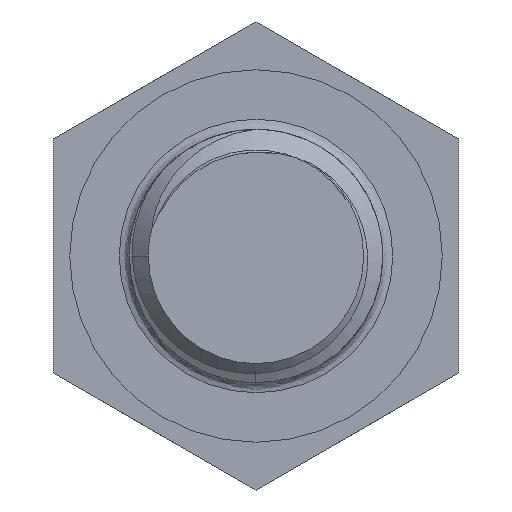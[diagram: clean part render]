
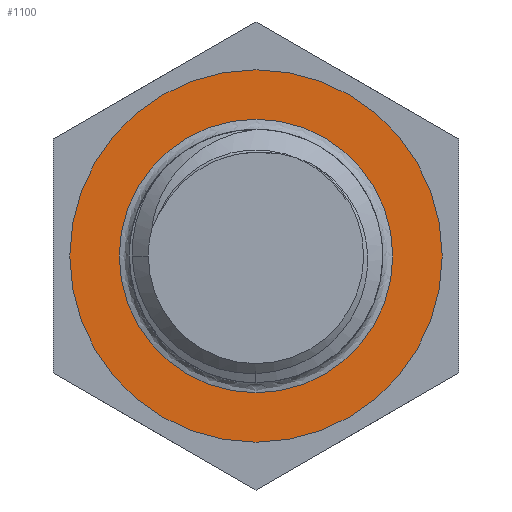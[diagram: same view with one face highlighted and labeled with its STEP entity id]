
A CAD part, left-side view. The second image highlights one B-rep face of the part: STEP entity #1100.
In plain terms, the highlighted planar face has unit normal (-1, 0, 0).
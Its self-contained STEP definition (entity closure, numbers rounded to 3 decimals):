
#817 = CYLINDRICAL_SURFACE('',#818,7.35);
#818 = AXIS2_PLACEMENT_3D('',#819,#820,#821);
#819 = CARTESIAN_POINT('',(-6.7,0.,0.));
#820 = DIRECTION('',(-1.,-0.,0.));
#821 = DIRECTION('',(0.,0.,-1.));
#1051 = VERTEX_POINT('',#1052);
#1052 = CARTESIAN_POINT('',(-7.,0.,-7.35));
#1073 = EDGE_CURVE('',#1051,#1051,#1074,.T.);
#1074 = SURFACE_CURVE('',#1075,(#1080,#1087),.PCURVE_S1.);
#1075 = CIRCLE('',#1076,7.35);
#1076 = AXIS2_PLACEMENT_3D('',#1077,#1078,#1079);
#1077 = CARTESIAN_POINT('',(-7.,0.,0.));
#1078 = DIRECTION('',(1.,-0.,0.));
#1079 = DIRECTION('',(0.,0.,-1.));
#1080 = PCURVE('',#817,#1081);
#1081 = DEFINITIONAL_REPRESENTATION('',(#1082),#1086);
#1082 = LINE('',#1083,#1084);
#1083 = CARTESIAN_POINT('',(-0.,0.3));
#1084 = VECTOR('',#1085,1.);
#1085 = DIRECTION('',(-1.,0.));
#1086 = ( GEOMETRIC_REPRESENTATION_CONTEXT(2) 
PARAMETRIC_REPRESENTATION_CONTEXT() REPRESENTATION_CONTEXT('2D SPACE',''
  ) );
#1087 = PCURVE('',#1088,#1093);
#1088 = PLANE('',#1089);
#1089 = AXIS2_PLACEMENT_3D('',#1090,#1091,#1092);
#1090 = CARTESIAN_POINT('',(-7.,0.,0.));
#1091 = DIRECTION('',(1.,0.,0.));
#1092 = DIRECTION('',(0.,0.,-1.));
#1093 = DEFINITIONAL_REPRESENTATION('',(#1094),#1098);
#1094 = CIRCLE('',#1095,7.35);
#1095 = AXIS2_PLACEMENT_2D('',#1096,#1097);
#1096 = CARTESIAN_POINT('',(0.,0.));
#1097 = DIRECTION('',(1.,0.));
#1098 = ( GEOMETRIC_REPRESENTATION_CONTEXT(2) 
PARAMETRIC_REPRESENTATION_CONTEXT() REPRESENTATION_CONTEXT('2D SPACE',''
  ) );
#1100 = ADVANCED_FACE('',(#1101,#1104),#1088,.F.);
#1101 = FACE_BOUND('',#1102,.F.);
#1102 = EDGE_LOOP('',(#1103));
#1103 = ORIENTED_EDGE('',*,*,#1073,.T.);
#1104 = FACE_BOUND('',#1105,.F.);
#1105 = EDGE_LOOP('',(#1106));
#1106 = ORIENTED_EDGE('',*,*,#1107,.F.);
#1107 = EDGE_CURVE('',#1108,#1108,#1110,.T.);
#1108 = VERTEX_POINT('',#1109);
#1109 = CARTESIAN_POINT('',(-7.,0.,-5.4));
#1110 = SURFACE_CURVE('',#1111,(#1116,#1123),.PCURVE_S1.);
#1111 = CIRCLE('',#1112,5.4);
#1112 = AXIS2_PLACEMENT_3D('',#1113,#1114,#1115);
#1113 = CARTESIAN_POINT('',(-7.,0.,0.));
#1114 = DIRECTION('',(1.,-0.,0.));
#1115 = DIRECTION('',(0.,0.,-1.));
#1116 = PCURVE('',#1088,#1117);
#1117 = DEFINITIONAL_REPRESENTATION('',(#1118),#1122);
#1118 = CIRCLE('',#1119,5.4);
#1119 = AXIS2_PLACEMENT_2D('',#1120,#1121);
#1120 = CARTESIAN_POINT('',(0.,0.));
#1121 = DIRECTION('',(1.,0.));
#1122 = ( GEOMETRIC_REPRESENTATION_CONTEXT(2) 
PARAMETRIC_REPRESENTATION_CONTEXT() REPRESENTATION_CONTEXT('2D SPACE',''
  ) );
#1123 = PCURVE('',#1124,#1133);
#1124 = SURFACE_OF_REVOLUTION('',#1125,#1130);
#1125 = CIRCLE('',#1126,0.4);
#1126 = AXIS2_PLACEMENT_3D('',#1127,#1128,#1129);
#1127 = CARTESIAN_POINT('',(-7.4,0.,-5.4));
#1128 = DIRECTION('',(0.,-1.,0.));
#1129 = DIRECTION('',(1.,0.,0.));
#1130 = AXIS1_PLACEMENT('',#1131,#1132);
#1131 = CARTESIAN_POINT('',(-7.,0.,0.));
#1132 = DIRECTION('',(1.,0.,0.));
#1133 = DEFINITIONAL_REPRESENTATION('',(#1134),#1138);
#1134 = LINE('',#1135,#1136);
#1135 = CARTESIAN_POINT('',(0.,0.));
#1136 = VECTOR('',#1137,1.);
#1137 = DIRECTION('',(1.,0.));
#1138 = ( GEOMETRIC_REPRESENTATION_CONTEXT(2) 
PARAMETRIC_REPRESENTATION_CONTEXT() REPRESENTATION_CONTEXT('2D SPACE',''
  ) );
